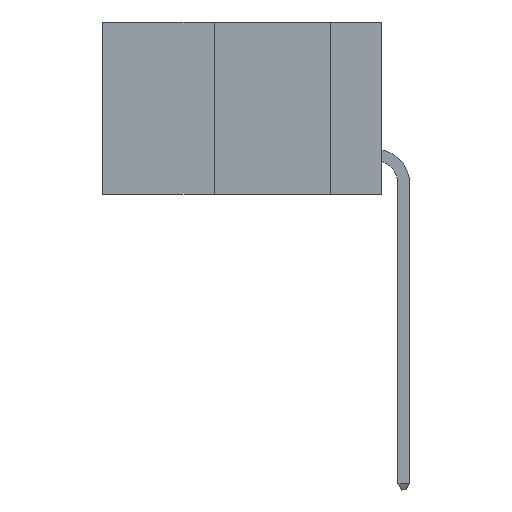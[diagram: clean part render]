
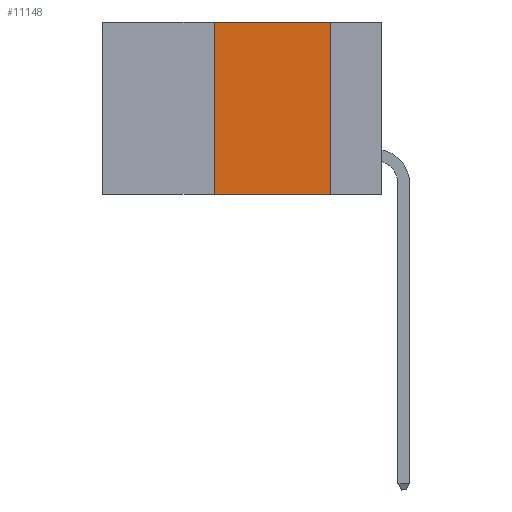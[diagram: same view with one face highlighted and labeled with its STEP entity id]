
A CAD part, left-side view. The second image highlights one B-rep face of the part: STEP entity #11148.
In plain terms, the highlighted planar face has unit normal (-1, 0, 0).
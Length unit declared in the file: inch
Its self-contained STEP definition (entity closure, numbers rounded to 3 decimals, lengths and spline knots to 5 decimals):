
#739 = ORIENTED_EDGE ( 'NONE', *, *, #9158, .F. ) ;
#1411 = DIRECTION ( 'NONE',  ( 0., -1., 0. ) ) ;
#1761 = VECTOR ( 'NONE', #1411, 39.37008 ) ;
#2252 = PLANE ( 'NONE',  #7447 ) ;
#2321 = CARTESIAN_POINT ( 'NONE',  ( 0., 0.6, -0.37 ) ) ;
#2331 = VERTEX_POINT ( 'NONE', #9497 ) ;
#2995 = CARTESIAN_POINT ( 'NONE',  ( 0., 0.36, 0. ) ) ;
#3020 = EDGE_LOOP ( 'NONE', ( #7809, #739, #8837, #4442 ) ) ;
#3763 = VECTOR ( 'NONE', #3781, 39.37008 ) ;
#3781 = DIRECTION ( 'NONE',  ( 0., -1., 0. ) ) ;
#4442 = ORIENTED_EDGE ( 'NONE', *, *, #10372, .T. ) ;
#4674 = DIRECTION ( 'NONE',  ( 1., 0., 0. ) ) ;
#5303 = VECTOR ( 'NONE', #6827, 39.37008 ) ;
#6082 = EDGE_CURVE ( 'NONE', #10555, #9446, #8128, .T. ) ;
#6388 = CARTESIAN_POINT ( 'NONE',  ( 0., 0.11, 0. ) ) ;
#6643 = CARTESIAN_POINT ( 'NONE',  ( 0., 0.6, 0. ) ) ;
#6827 = DIRECTION ( 'NONE',  ( 0., 0., 1. ) ) ;
#7045 = DIRECTION ( 'NONE',  ( 0., 0., -1. ) ) ;
#7369 = VECTOR ( 'NONE', #7045, 39.37008 ) ;
#7447 = AXIS2_PLACEMENT_3D ( 'NONE', #10523, #4674, #11504 ) ;
#7546 = FACE_OUTER_BOUND ( 'NONE', #3020, .T. ) ;
#7809 = ORIENTED_EDGE ( 'NONE', *, *, #6082, .F. ) ;
#7879 = EDGE_CURVE ( 'NONE', #12384, #2331, #8542, .T. ) ;
#8128 = LINE ( 'NONE', #12034, #7369 ) ;
#8542 = LINE ( 'NONE', #2995, #5303 ) ;
#8837 = ORIENTED_EDGE ( 'NONE', *, *, #7879, .F. ) ;
#9158 = EDGE_CURVE ( 'NONE', #2331, #10555, #11553, .T. ) ;
#9446 = VERTEX_POINT ( 'NONE', #11184 ) ;
#9497 = CARTESIAN_POINT ( 'NONE',  ( 0., 0.36, 0. ) ) ;
#10372 = EDGE_CURVE ( 'NONE', #12384, #9446, #11377, .T. ) ;
#10523 = CARTESIAN_POINT ( 'NONE',  ( 0., 0.6, 0. ) ) ;
#10555 = VERTEX_POINT ( 'NONE', #6388 ) ;
#10582 = CARTESIAN_POINT ( 'NONE',  ( 0., 0.36, -0.37 ) ) ;
#11148 = ADVANCED_FACE ( 'NONE', ( #7546 ), #2252, .F. ) ;
#11184 = CARTESIAN_POINT ( 'NONE',  ( 0., 0.11, -0.37 ) ) ;
#11377 = LINE ( 'NONE', #2321, #1761 ) ;
#11504 = DIRECTION ( 'NONE',  ( 0., 0., -1. ) ) ;
#11553 = LINE ( 'NONE', #6643, #3763 ) ;
#12034 = CARTESIAN_POINT ( 'NONE',  ( 0., 0.11, 0. ) ) ;
#12384 = VERTEX_POINT ( 'NONE', #10582 ) ;
